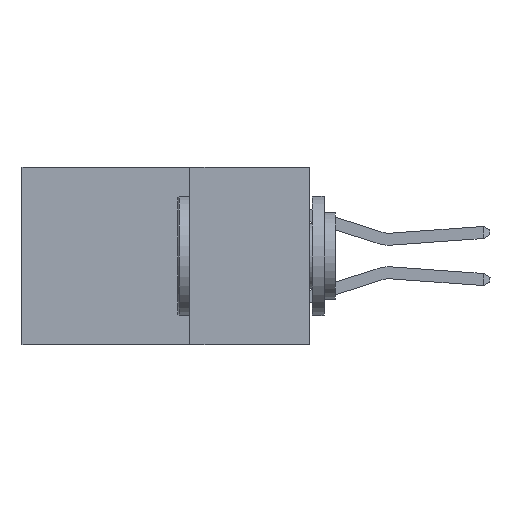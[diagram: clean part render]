
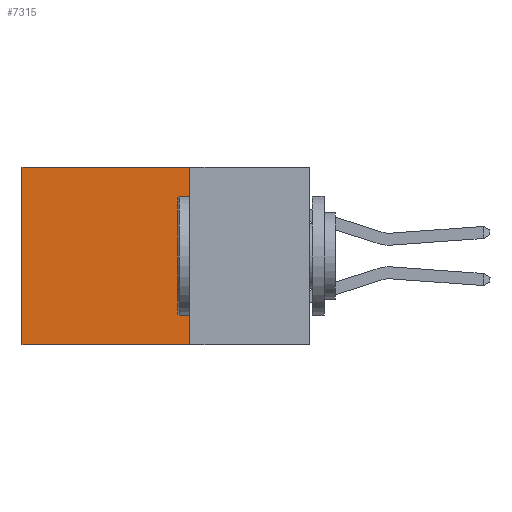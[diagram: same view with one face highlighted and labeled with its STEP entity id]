
A CAD part, left-side view. The second image highlights one B-rep face of the part: STEP entity #7315.
In plain terms, the highlighted planar face has unit normal (-1, 0, 0).
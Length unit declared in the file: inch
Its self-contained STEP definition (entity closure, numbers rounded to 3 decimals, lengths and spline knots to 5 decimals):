
#859 = LINE ( 'NONE', #9579, #12486 ) ;
#995 = DIRECTION ( 'NONE',  ( 1., 0., 0. ) ) ;
#1058 = PLANE ( 'NONE',  #5480 ) ;
#1624 = EDGE_CURVE ( 'NONE', #2811, #16165, #7272, .T. ) ;
#1639 = DIRECTION ( 'NONE',  ( 0., 0., -1. ) ) ;
#2439 = CARTESIAN_POINT ( 'NONE',  ( 0.2615, 0.25, -0.37 ) ) ;
#2811 = VERTEX_POINT ( 'NONE', #17744 ) ;
#3817 = LINE ( 'NONE', #15301, #11730 ) ;
#4046 = DIRECTION ( 'NONE',  ( 0., 0., -1. ) ) ;
#4378 = ORIENTED_EDGE ( 'NONE', *, *, #1624, .F. ) ;
#5480 = AXIS2_PLACEMENT_3D ( 'NONE', #2439, #995, #4046 ) ;
#5823 = CARTESIAN_POINT ( 'NONE',  ( 0.2615, 0.6, -0.37 ) ) ;
#6385 = EDGE_CURVE ( 'NONE', #6962, #12857, #3817, .T. ) ;
#6962 = VERTEX_POINT ( 'NONE', #18604 ) ;
#7053 = DIRECTION ( 'NONE',  ( 0., 0., -1. ) ) ;
#7272 = LINE ( 'NONE', #14967, #18997 ) ;
#7315 = ADVANCED_FACE ( 'NONE', ( #19223 ), #1058, .F. ) ;
#8160 = CARTESIAN_POINT ( 'NONE',  ( 0.2615, 0.6, 0. ) ) ;
#8360 = LINE ( 'NONE', #17810, #20008 ) ;
#9579 = CARTESIAN_POINT ( 'NONE',  ( 0.2615, 0.25, -0.37 ) ) ;
#10559 = EDGE_CURVE ( 'NONE', #12857, #16165, #8360, .T. ) ;
#11006 = EDGE_CURVE ( 'NONE', #6962, #2811, #859, .T. ) ;
#11381 = ORIENTED_EDGE ( 'NONE', *, *, #10559, .T. ) ;
#11447 = DIRECTION ( 'NONE',  ( 0., 1., 0. ) ) ;
#11730 = VECTOR ( 'NONE', #11447, 39.37008 ) ;
#12486 = VECTOR ( 'NONE', #1639, 39.37008 ) ;
#12730 = ORIENTED_EDGE ( 'NONE', *, *, #6385, .T. ) ;
#12857 = VERTEX_POINT ( 'NONE', #8160 ) ;
#14967 = CARTESIAN_POINT ( 'NONE',  ( 0.2615, 0.25, -0.37 ) ) ;
#15301 = CARTESIAN_POINT ( 'NONE',  ( 0.2615, 0.25, 0. ) ) ;
#16165 = VERTEX_POINT ( 'NONE', #5823 ) ;
#17324 = ORIENTED_EDGE ( 'NONE', *, *, #11006, .F. ) ;
#17744 = CARTESIAN_POINT ( 'NONE',  ( 0.2615, 0.25, -0.37 ) ) ;
#17810 = CARTESIAN_POINT ( 'NONE',  ( 0.2615, 0.6, -0.37 ) ) ;
#18031 = DIRECTION ( 'NONE',  ( 0., 1., 0. ) ) ;
#18604 = CARTESIAN_POINT ( 'NONE',  ( 0.2615, 0.25, 0. ) ) ;
#18997 = VECTOR ( 'NONE', #18031, 39.37008 ) ;
#19223 = FACE_OUTER_BOUND ( 'NONE', #19360, .T. ) ;
#19360 = EDGE_LOOP ( 'NONE', ( #11381, #4378, #17324, #12730 ) ) ;
#20008 = VECTOR ( 'NONE', #7053, 39.37008 ) ;
